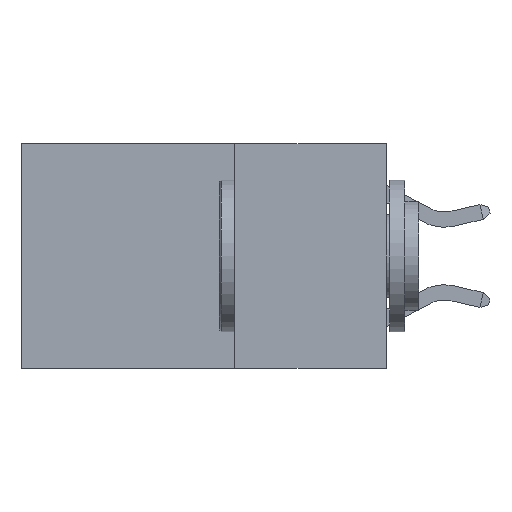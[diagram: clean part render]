
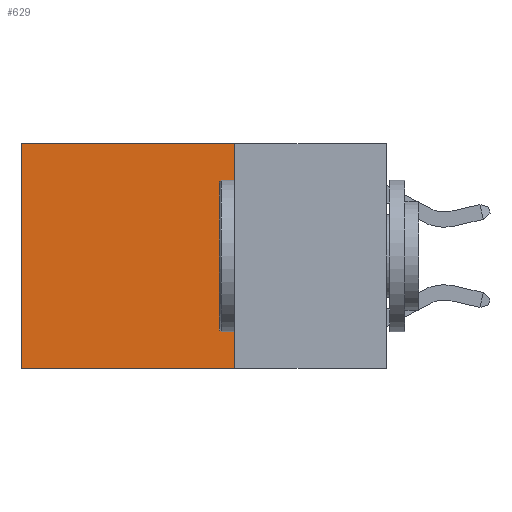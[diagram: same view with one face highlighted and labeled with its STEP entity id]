
A CAD part, left-side view. The second image highlights one B-rep face of the part: STEP entity #629.
In plain terms, the highlighted planar face has unit normal (-1, 0, 0).
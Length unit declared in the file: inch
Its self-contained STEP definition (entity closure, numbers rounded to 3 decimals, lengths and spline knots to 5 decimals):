
#135 = VECTOR ( 'NONE', #5491, 39.37008 ) ;
#136 = CARTESIAN_POINT ( 'NONE',  ( 0.2625, 0.6, -0.37 ) ) ;
#236 = VERTEX_POINT ( 'NONE', #9445 ) ;
#457 = CARTESIAN_POINT ( 'NONE',  ( 0.2625, 0.6, 0. ) ) ;
#534 = AXIS2_PLACEMENT_3D ( 'NONE', #10546, #6639, #10382 ) ;
#629 = ADVANCED_FACE ( 'NONE', ( #1288 ), #7006, .F. ) ;
#765 = ORIENTED_EDGE ( 'NONE', *, *, #8431, .F. ) ;
#1288 = FACE_OUTER_BOUND ( 'NONE', #8132, .T. ) ;
#2078 = DIRECTION ( 'NONE',  ( 0., 1., 0. ) ) ;
#2589 = EDGE_CURVE ( 'NONE', #236, #6794, #2836, .T. ) ;
#2836 = LINE ( 'NONE', #7112, #6782 ) ;
#2899 = ORIENTED_EDGE ( 'NONE', *, *, #3426, .T. ) ;
#3426 = EDGE_CURVE ( 'NONE', #236, #6219, #9129, .T. ) ;
#3745 = LINE ( 'NONE', #9702, #8172 ) ;
#5491 = DIRECTION ( 'NONE',  ( 0., 1., 0. ) ) ;
#6219 = VERTEX_POINT ( 'NONE', #457 ) ;
#6639 = DIRECTION ( 'NONE',  ( 1., 0., 0. ) ) ;
#6670 = VERTEX_POINT ( 'NONE', #136 ) ;
#6782 = VECTOR ( 'NONE', #6835, 39.37008 ) ;
#6794 = VERTEX_POINT ( 'NONE', #10155 ) ;
#6835 = DIRECTION ( 'NONE',  ( 0., 0., -1. ) ) ;
#6900 = LINE ( 'NONE', #9514, #135 ) ;
#7006 = PLANE ( 'NONE',  #534 ) ;
#7024 = VECTOR ( 'NONE', #2078, 39.37008 ) ;
#7112 = CARTESIAN_POINT ( 'NONE',  ( 0.2625, 0.25, 0. ) ) ;
#7244 = ORIENTED_EDGE ( 'NONE', *, *, #7849, .T. ) ;
#7849 = EDGE_CURVE ( 'NONE', #6219, #6670, #3745, .T. ) ;
#8132 = EDGE_LOOP ( 'NONE', ( #7244, #765, #8480, #2899 ) ) ;
#8172 = VECTOR ( 'NONE', #10489, 39.37008 ) ;
#8431 = EDGE_CURVE ( 'NONE', #6794, #6670, #6900, .T. ) ;
#8480 = ORIENTED_EDGE ( 'NONE', *, *, #2589, .F. ) ;
#9129 = LINE ( 'NONE', #10254, #7024 ) ;
#9445 = CARTESIAN_POINT ( 'NONE',  ( 0.2625, 0.25, 0. ) ) ;
#9514 = CARTESIAN_POINT ( 'NONE',  ( 0.2625, 0.25, -0.37 ) ) ;
#9702 = CARTESIAN_POINT ( 'NONE',  ( 0.2625, 0.6, 0. ) ) ;
#10155 = CARTESIAN_POINT ( 'NONE',  ( 0.2625, 0.25, -0.37 ) ) ;
#10254 = CARTESIAN_POINT ( 'NONE',  ( 0.2625, 0.25, 0. ) ) ;
#10382 = DIRECTION ( 'NONE',  ( 0., 0., -1. ) ) ;
#10489 = DIRECTION ( 'NONE',  ( 0., 0., -1. ) ) ;
#10546 = CARTESIAN_POINT ( 'NONE',  ( 0.2625, 0.25, 0. ) ) ;
